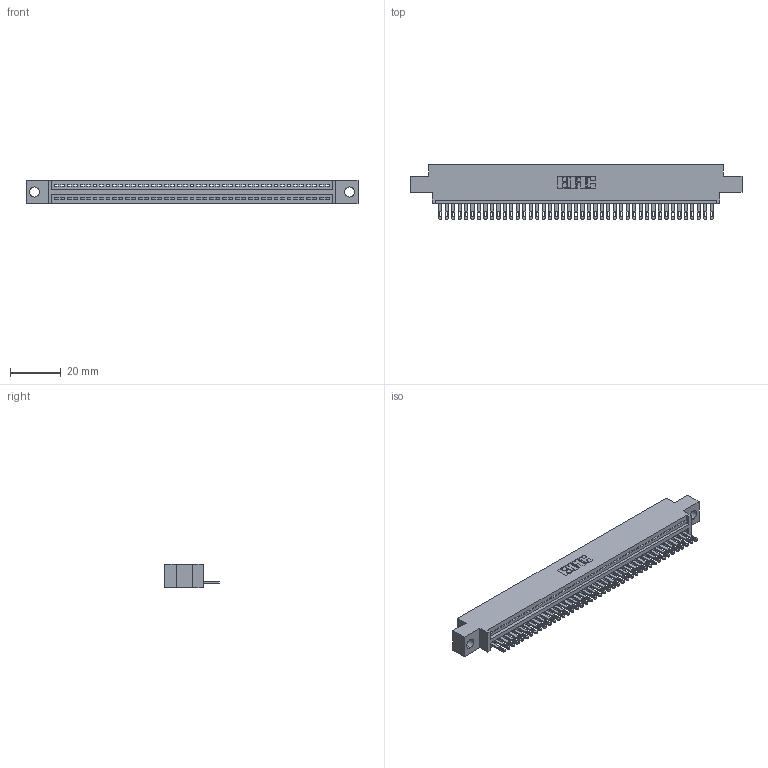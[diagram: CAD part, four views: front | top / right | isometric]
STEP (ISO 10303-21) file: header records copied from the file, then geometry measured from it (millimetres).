
FILE_DESCRIPTION (( 'STEP AP203' ), '1' );
FILE_NAME ('895-043-500-604.STEP', '2020-09-27T02:15:53', ( '' ), ( '' ), 'SwSTEP 2.0', 'SolidWorks 2020', '' );
FILE_SCHEMA (( 'CONFIG_CONTROL_DESIGN' ));
Length unit declared in the file: inch
Products named in the file (3): 895-043-500-604; 845 Part_0.170 Offset - 0.156 Dia-TH; 345-292-001_345-293-100
Assembly tree (44 placements, depth 2):
  895-043-500-604
    845 Part_0.170 Offset - 0.156 Dia-TH
    345-292-001_345-293-100  x43
Bounding box: 130.43 x 21.51 x 9.4 mm (x, y, z)
Volume: 12221.8 mm3; surface area: 16287.2 mm2
Topology: 44 solids, 44 shells, 2452 faces, 7577 edges, 5050 vertices
Faces by surface type: plane 1546, cylinder 906
Entity records: 32293 total; most frequent: CARTESIAN_POINT 5601, ORIENTED_EDGE 5578, DIRECTION 4891, EDGE_CURVE 2789, LINE 2481, VECTOR 2481, VERTEX_POINT 1858, AXIS2_PLACEMENT_3D 1205
